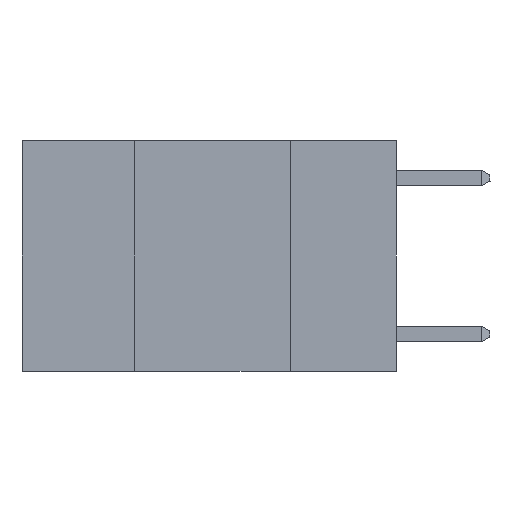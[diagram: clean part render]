
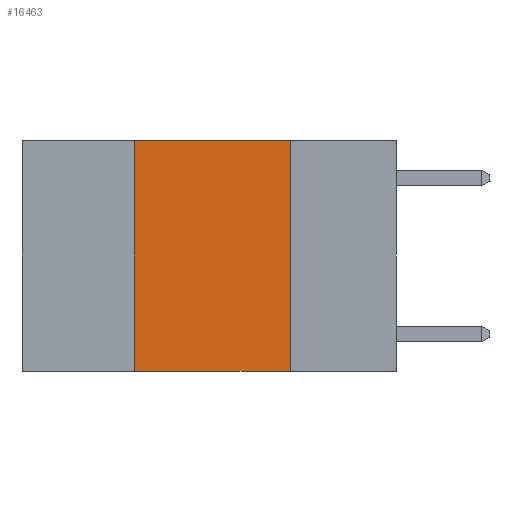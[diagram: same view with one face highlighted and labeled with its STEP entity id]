
A CAD part, left-side view. The second image highlights one B-rep face of the part: STEP entity #16463.
In plain terms, the highlighted planar face has unit normal (-1, 0, 0).
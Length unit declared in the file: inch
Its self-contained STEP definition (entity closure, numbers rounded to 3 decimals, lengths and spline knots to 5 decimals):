
#66 = VERTEX_POINT ( 'NONE', #8654 ) ;
#234 = DIRECTION ( 'NONE',  ( 0., -1., 0. ) ) ;
#269 = ORIENTED_EDGE ( 'NONE', *, *, #12610, .T. ) ;
#401 = CARTESIAN_POINT ( 'NONE',  ( 0., 0.6, -0.37 ) ) ;
#1107 = ORIENTED_EDGE ( 'NONE', *, *, #17684, .F. ) ;
#1389 = LINE ( 'NONE', #11157, #17874 ) ;
#1485 = PLANE ( 'NONE',  #8437 ) ;
#1645 = CARTESIAN_POINT ( 'NONE',  ( 0., 0.17, 0. ) ) ;
#1736 = ORIENTED_EDGE ( 'NONE', *, *, #15883, .F. ) ;
#1914 = FACE_OUTER_BOUND ( 'NONE', #15174, .T. ) ;
#4533 = DIRECTION ( 'NONE',  ( 1., 0., 0. ) ) ;
#7110 = LINE ( 'NONE', #401, #11348 ) ;
#8437 = AXIS2_PLACEMENT_3D ( 'NONE', #15450, #4533, #15523 ) ;
#8654 = CARTESIAN_POINT ( 'NONE',  ( 0., 0.17, -0.37 ) ) ;
#9578 = VECTOR ( 'NONE', #11851, 39.37008 ) ;
#11157 = CARTESIAN_POINT ( 'NONE',  ( 0., 0.42, 0. ) ) ;
#11348 = VECTOR ( 'NONE', #18769, 39.37008 ) ;
#11851 = DIRECTION ( 'NONE',  ( 0., 0., -1. ) ) ;
#12197 = ORIENTED_EDGE ( 'NONE', *, *, #16685, .F. ) ;
#12410 = VERTEX_POINT ( 'NONE', #17076 ) ;
#12610 = EDGE_CURVE ( 'NONE', #16196, #66, #7110, .T. ) ;
#14630 = LINE ( 'NONE', #18473, #18188 ) ;
#15174 = EDGE_LOOP ( 'NONE', ( #12197, #1736, #1107, #269 ) ) ;
#15450 = CARTESIAN_POINT ( 'NONE',  ( 0., 0.6, 0. ) ) ;
#15523 = DIRECTION ( 'NONE',  ( 0., 0., -1. ) ) ;
#15883 = EDGE_CURVE ( 'NONE', #12410, #15962, #14630, .T. ) ;
#15962 = VERTEX_POINT ( 'NONE', #1645 ) ;
#16196 = VERTEX_POINT ( 'NONE', #19190 ) ;
#16463 = ADVANCED_FACE ( 'NONE', ( #1914 ), #1485, .F. ) ;
#16685 = EDGE_CURVE ( 'NONE', #15962, #66, #17232, .T. ) ;
#17076 = CARTESIAN_POINT ( 'NONE',  ( 0., 0.42, 0. ) ) ;
#17201 = DIRECTION ( 'NONE',  ( 0., 0., 1. ) ) ;
#17232 = LINE ( 'NONE', #17876, #9578 ) ;
#17684 = EDGE_CURVE ( 'NONE', #16196, #12410, #1389, .T. ) ;
#17874 = VECTOR ( 'NONE', #17201, 39.37008 ) ;
#17876 = CARTESIAN_POINT ( 'NONE',  ( 0., 0.17, 0. ) ) ;
#18188 = VECTOR ( 'NONE', #234, 39.37008 ) ;
#18473 = CARTESIAN_POINT ( 'NONE',  ( 0., 0.6, 0. ) ) ;
#18769 = DIRECTION ( 'NONE',  ( 0., -1., 0. ) ) ;
#19190 = CARTESIAN_POINT ( 'NONE',  ( 0., 0.42, -0.37 ) ) ;
